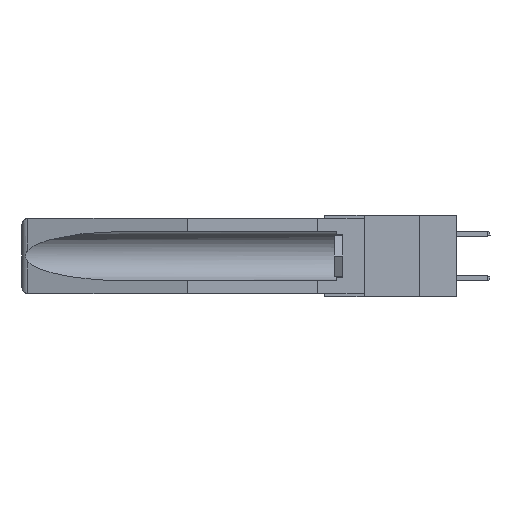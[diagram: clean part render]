
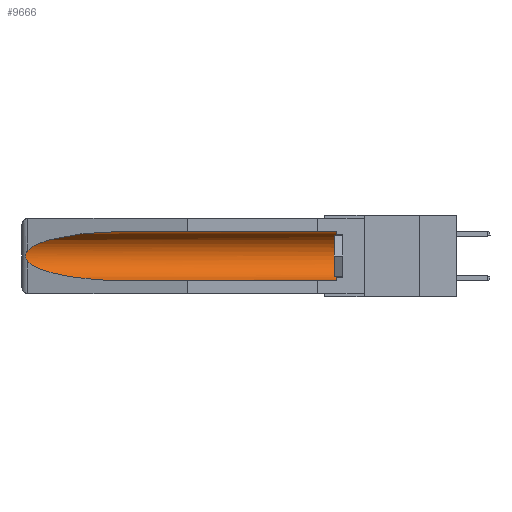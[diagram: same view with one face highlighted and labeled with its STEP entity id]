
A CAD part, left-side view. The second image highlights one B-rep face of the part: STEP entity #9666.
In plain terms, the highlighted cylindrical face has radius 2.857 mm (diameter 5.715 mm), a partial arc.
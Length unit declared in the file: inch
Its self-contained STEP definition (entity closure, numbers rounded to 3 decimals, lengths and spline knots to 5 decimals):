
#247 = CARTESIAN_POINT ( 'NONE',  ( 0.155, 0.126, -0.1715 ) ) ;
#1417 = CARTESIAN_POINT ( 'NONE',  ( 0.155, 1.07973, -0.059 ) ) ;
#1526 = VECTOR ( 'NONE', #20109, 39.37008 ) ;
#1961 = CARTESIAN_POINT ( 'NONE',  ( 0.21114, 1.30732, -0.059 ) ) ;
#1999 = ORIENTED_EDGE ( 'NONE', *, *, #24168, .T. ) ;
#2455 = CARTESIAN_POINT ( 'NONE',  ( 0.21114, 1.30732, -0.284 ) ) ;
#2870 = CARTESIAN_POINT ( 'NONE',  ( 0.26537, 1.52718, -0.14972 ) ) ;
#3041 = CIRCLE ( 'NONE', #25262, 0.1125 ) ;
#4213 = VERTEX_POINT ( 'NONE', #19897 ) ;
#4891 = CARTESIAN_POINT ( 'NONE',  ( 0.26597, 1.52961, -0.15275 ) ) ;
#5330 = CARTESIAN_POINT ( 'NONE',  ( 0.26655, 1.53094, -0.18657 ) ) ;
#6129 = DIRECTION ( 'NONE',  ( 0., 1., 0. ) ) ;
#6665 = EDGE_CURVE ( 'NONE', #6924, #9988, #3041, .T. ) ;
#6675 = CARTESIAN_POINT ( 'NONE',  ( 0.155, 1.07973, -0.284 ) ) ;
#6745 = VECTOR ( 'NONE', #6129, 39.37008 ) ;
#6924 = VERTEX_POINT ( 'NONE', #15452 ) ;
#6998 = ORIENTED_EDGE ( 'NONE', *, *, #17219, .T. ) ;
#7876 = CARTESIAN_POINT ( 'NONE',  ( 0.155, 1.07973, -0.059 ) ) ;
#8176 = LINE ( 'NONE', #17895, #1526 ) ;
#8253 = CARTESIAN_POINT ( 'NONE',  ( 0.155, -0.30754, -0.284 ) ) ;
#8325 = VERTEX_POINT ( 'NONE', #6675 ) ;
#8442 = EDGE_CURVE ( 'NONE', #18862, #4213, #11739, .T. ) ;
#8693 = CYLINDRICAL_SURFACE ( 'NONE', #16508, 0.1125 ) ;
#9215 = CARTESIAN_POINT ( 'NONE',  ( 0.2673, 1.5327, -0.16383 ) ) ;
#9666 = ADVANCED_FACE ( 'NONE', ( #10284 ), #8693, .F. ) ;
#9899 = DIRECTION ( 'NONE',  ( 0., 0., 1. ) ) ;
#9988 = VERTEX_POINT ( 'NONE', #25796 ) ;
#10092 = ORIENTED_EDGE ( 'NONE', *, *, #6665, .T. ) ;
#10284 = FACE_OUTER_BOUND ( 'NONE', #23039, .T. ) ;
#10298 = DIRECTION ( 'NONE',  ( 0., -1., 0. ) ) ;
#10395 = DIRECTION ( 'NONE',  ( 0., 0., 1. ) ) ;
#11161 = CARTESIAN_POINT ( 'NONE',  ( 0.26537, 1.52718, -0.14972 ) ) ;
#11739 = B_SPLINE_CURVE_WITH_KNOTS ( 'NONE', 3,
 ( #2870, #4891, #21566, #9215, #23337, #15552, #17410, #5330, #17228, #19262 ),
 .UNSPECIFIED., .F., .F.,
 ( 4, 2, 2, 2, 4 ),
 ( 0., 0.00029, 0.00058, 0.00087, 0.00117 ),
 .UNSPECIFIED. ) ;
#15232 = LINE ( 'NONE', #8253, #6745 ) ;
#15452 = CARTESIAN_POINT ( 'NONE',  ( 0.155, 0.126, -0.284 ) ) ;
#15552 = CARTESIAN_POINT ( 'NONE',  ( 0.2675, 1.53308, -0.17534 ) ) ;
#15701 = CARTESIAN_POINT ( 'NONE',  ( 0.155, -0.30754, -0.1715 ) ) ;
#15969 = CARTESIAN_POINT ( 'NONE',  ( 0.25451, 1.48313, -0.09465 ) ) ;
#16487 = VERTEX_POINT ( 'NONE', #1417 ) ;
#16508 = AXIS2_PLACEMENT_3D ( 'NONE', #15701, #25784, #9899 ) ;
#17219 = EDGE_CURVE ( 'NONE', #16487, #18862, #24546, .T. ) ;
#17228 = CARTESIAN_POINT ( 'NONE',  ( 0.26597, 1.5296, -0.19026 ) ) ;
#17410 = CARTESIAN_POINT ( 'NONE',  ( 0.2673, 1.53269, -0.17917 ) ) ;
#17895 = CARTESIAN_POINT ( 'NONE',  ( 0.155, -0.30754, -0.059 ) ) ;
#18862 = VERTEX_POINT ( 'NONE', #11161 ) ;
#19262 = CARTESIAN_POINT ( 'NONE',  ( 0.26537, 1.52718, -0.19328 ) ) ;
#19668 = ORIENTED_EDGE ( 'NONE', *, *, #20150, .F. ) ;
#19827 =( BOUNDED_CURVE ( )  B_SPLINE_CURVE ( 3, ( #22425, #20643, #2455, #20723 ),
 .UNSPECIFIED., .F., .F. ) 
 B_SPLINE_CURVE_WITH_KNOTS ( ( 4, 4 ),
 ( 0.1948, 1.5708 ),
 .UNSPECIFIED. ) 
 CURVE ( )  GEOMETRIC_REPRESENTATION_ITEM ( )  RATIONAL_B_SPLINE_CURVE ( ( 1., 0.848, 0.848, 1. ) ) 
 REPRESENTATION_ITEM ( '' )  );
#19897 = CARTESIAN_POINT ( 'NONE',  ( 0.26537, 1.52718, -0.19328 ) ) ;
#20109 = DIRECTION ( 'NONE',  ( 0., 1., 0. ) ) ;
#20129 = CARTESIAN_POINT ( 'NONE',  ( 0.26537, 1.52718, -0.14972 ) ) ;
#20150 = EDGE_CURVE ( 'NONE', #6924, #8325, #15232, .T. ) ;
#20643 = CARTESIAN_POINT ( 'NONE',  ( 0.25451, 1.48313, -0.24835 ) ) ;
#20723 = CARTESIAN_POINT ( 'NONE',  ( 0.155, 1.07973, -0.284 ) ) ;
#20832 = EDGE_CURVE ( 'NONE', #9988, #16487, #8176, .T. ) ;
#21379 = ORIENTED_EDGE ( 'NONE', *, *, #8442, .T. ) ;
#21566 = CARTESIAN_POINT ( 'NONE',  ( 0.26654, 1.53092, -0.15636 ) ) ;
#22425 = CARTESIAN_POINT ( 'NONE',  ( 0.26537, 1.52718, -0.19328 ) ) ;
#23039 = EDGE_LOOP ( 'NONE', ( #6998, #21379, #1999, #19668, #10092, #23376 ) ) ;
#23337 = CARTESIAN_POINT ( 'NONE',  ( 0.2675, 1.53308, -0.16763 ) ) ;
#23376 = ORIENTED_EDGE ( 'NONE', *, *, #20832, .T. ) ;
#24168 = EDGE_CURVE ( 'NONE', #4213, #8325, #19827, .T. ) ;
#24546 =( BOUNDED_CURVE ( )  B_SPLINE_CURVE ( 3, ( #7876, #1961, #15969, #20129 ),
 .UNSPECIFIED., .F., .F. ) 
 B_SPLINE_CURVE_WITH_KNOTS ( ( 4, 4 ),
 ( 4.71239, 6.08839 ),
 .UNSPECIFIED. ) 
 CURVE ( )  GEOMETRIC_REPRESENTATION_ITEM ( )  RATIONAL_B_SPLINE_CURVE ( ( 1., 0.848, 0.848, 1. ) ) 
 REPRESENTATION_ITEM ( '' )  );
#25262 = AXIS2_PLACEMENT_3D ( 'NONE', #247, #10298, #10395 ) ;
#25784 = DIRECTION ( 'NONE',  ( 0., 1., 0. ) ) ;
#25796 = CARTESIAN_POINT ( 'NONE',  ( 0.155, 0.126, -0.059 ) ) ;
